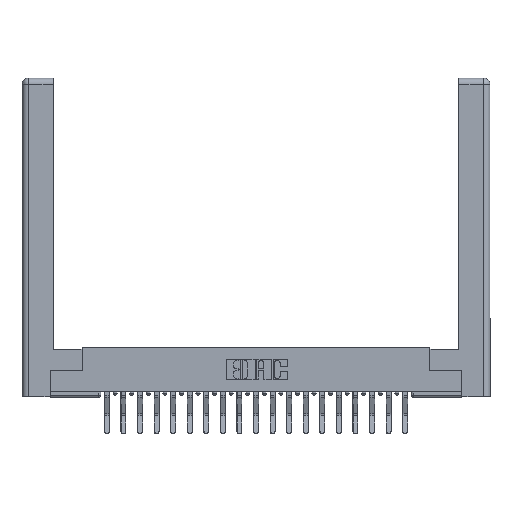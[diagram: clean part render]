
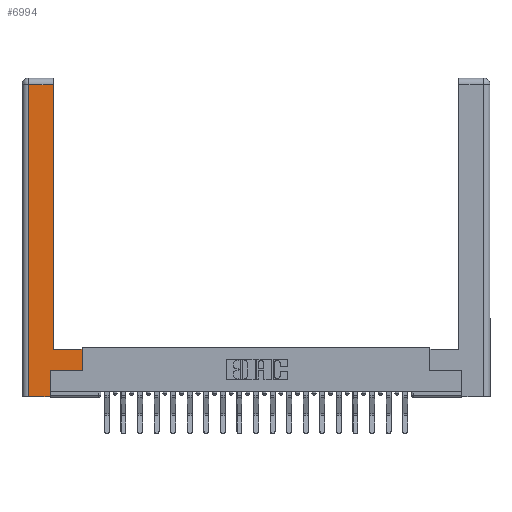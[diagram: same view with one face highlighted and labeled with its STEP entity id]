
A CAD part, top view. The second image highlights one B-rep face of the part: STEP entity #6994.
In plain terms, the highlighted planar face has unit normal (0, 0, 1).
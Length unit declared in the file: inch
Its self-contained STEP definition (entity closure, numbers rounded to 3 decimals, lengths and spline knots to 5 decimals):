
#736 = CARTESIAN_POINT ( 'NONE',  ( 0.565, 0.245, 0. ) ) ;
#1228 = VECTOR ( 'NONE', #2100, 39.37008 ) ;
#1579 = CARTESIAN_POINT ( 'NONE',  ( 0.0615, 2.94, 0. ) ) ;
#1659 = AXIS2_PLACEMENT_3D ( 'NONE', #2252, #16117, #19521 ) ;
#1667 = CARTESIAN_POINT ( 'NONE',  ( 0.295, 0.45, 0. ) ) ;
#1779 = VERTEX_POINT ( 'NONE', #20524 ) ;
#2100 = DIRECTION ( 'NONE',  ( 0., 1., 0. ) ) ;
#2252 = CARTESIAN_POINT ( 'NONE',  ( 0., 0., 0. ) ) ;
#2592 = LINE ( 'NONE', #6267, #15879 ) ;
#3101 = CARTESIAN_POINT ( 'NONE',  ( 0.295, 2.94, 0. ) ) ;
#3472 = DIRECTION ( 'NONE',  ( -1., 0., 0. ) ) ;
#4064 = CARTESIAN_POINT ( 'NONE',  ( 0.565, 0.45, 0. ) ) ;
#4381 = EDGE_CURVE ( 'NONE', #16245, #14861, #12408, .T. ) ;
#4426 = LINE ( 'NONE', #10451, #22373 ) ;
#5362 = VECTOR ( 'NONE', #15289, 39.37008 ) ;
#5821 = DIRECTION ( 'NONE',  ( 0., 1., 0. ) ) ;
#5890 = VECTOR ( 'NONE', #5821, 39.37008 ) ;
#5958 = VECTOR ( 'NONE', #19146, 39.37008 ) ;
#6267 = CARTESIAN_POINT ( 'NONE',  ( 0.0615, 0., 0. ) ) ;
#6269 = VERTEX_POINT ( 'NONE', #3101 ) ;
#6994 = ADVANCED_FACE ( 'NONE', ( #21764 ), #12651, .F. ) ;
#8151 = ORIENTED_EDGE ( 'NONE', *, *, #16688, .T. ) ;
#8344 = LINE ( 'NONE', #736, #18120 ) ;
#9916 = LINE ( 'NONE', #14165, #1228 ) ;
#10451 = CARTESIAN_POINT ( 'NONE',  ( 0.0615, 2.94, 0. ) ) ;
#10456 = DIRECTION ( 'NONE',  ( -1., 0., 0. ) ) ;
#10518 = CARTESIAN_POINT ( 'NONE',  ( 0.295, 0.45, 0. ) ) ;
#11649 = ORIENTED_EDGE ( 'NONE', *, *, #18595, .T. ) ;
#12361 = ORIENTED_EDGE ( 'NONE', *, *, #20280, .T. ) ;
#12408 = LINE ( 'NONE', #4064, #5890 ) ;
#12465 = VERTEX_POINT ( 'NONE', #12523 ) ;
#12523 = CARTESIAN_POINT ( 'NONE',  ( 0.0615, 0., 0. ) ) ;
#12590 = EDGE_CURVE ( 'NONE', #16413, #16245, #8344, .T. ) ;
#12651 = PLANE ( 'NONE',  #1659 ) ;
#13874 = LINE ( 'NONE', #1667, #21977 ) ;
#14165 = CARTESIAN_POINT ( 'NONE',  ( 0.265, 0.245, 0. ) ) ;
#14385 = EDGE_LOOP ( 'NONE', ( #8151, #12361, #11649, #19383, #17170, #17784, #17348, #18415 ) ) ;
#14861 = VERTEX_POINT ( 'NONE', #21602 ) ;
#15128 = EDGE_CURVE ( 'NONE', #14861, #22238, #13874, .T. ) ;
#15289 = DIRECTION ( 'NONE',  ( 0., 1., 0. ) ) ;
#15859 = CARTESIAN_POINT ( 'NONE',  ( 0.265, 0.245, 0. ) ) ;
#15879 = VECTOR ( 'NONE', #17947, 39.37008 ) ;
#16117 = DIRECTION ( 'NONE',  ( 0., 0., -1. ) ) ;
#16245 = VERTEX_POINT ( 'NONE', #22091 ) ;
#16277 = LINE ( 'NONE', #20738, #5958 ) ;
#16413 = VERTEX_POINT ( 'NONE', #15859 ) ;
#16688 = EDGE_CURVE ( 'NONE', #22238, #6269, #19211, .T. ) ;
#16985 = VERTEX_POINT ( 'NONE', #1579 ) ;
#17170 = ORIENTED_EDGE ( 'NONE', *, *, #19042, .T. ) ;
#17348 = ORIENTED_EDGE ( 'NONE', *, *, #4381, .T. ) ;
#17784 = ORIENTED_EDGE ( 'NONE', *, *, #12590, .T. ) ;
#17947 = DIRECTION ( 'NONE',  ( 0., -1., 0. ) ) ;
#18120 = VECTOR ( 'NONE', #19844, 39.37008 ) ;
#18415 = ORIENTED_EDGE ( 'NONE', *, *, #15128, .T. ) ;
#18595 = EDGE_CURVE ( 'NONE', #16985, #12465, #2592, .T. ) ;
#19042 = EDGE_CURVE ( 'NONE', #1779, #16413, #9916, .T. ) ;
#19146 = DIRECTION ( 'NONE',  ( 1., 0., 0. ) ) ;
#19211 = LINE ( 'NONE', #22190, #5362 ) ;
#19383 = ORIENTED_EDGE ( 'NONE', *, *, #22236, .T. ) ;
#19521 = DIRECTION ( 'NONE',  ( -1., 0., 0. ) ) ;
#19844 = DIRECTION ( 'NONE',  ( 1., 0., 0. ) ) ;
#20280 = EDGE_CURVE ( 'NONE', #6269, #16985, #4426, .T. ) ;
#20524 = CARTESIAN_POINT ( 'NONE',  ( 0.265, 0., 0. ) ) ;
#20738 = CARTESIAN_POINT ( 'NONE',  ( 0.265, 0., 0. ) ) ;
#21602 = CARTESIAN_POINT ( 'NONE',  ( 0.565, 0.45, 0. ) ) ;
#21764 = FACE_OUTER_BOUND ( 'NONE', #14385, .T. ) ;
#21977 = VECTOR ( 'NONE', #10456, 39.37008 ) ;
#22091 = CARTESIAN_POINT ( 'NONE',  ( 0.565, 0.245, 0. ) ) ;
#22190 = CARTESIAN_POINT ( 'NONE',  ( 0.295, 3., 0. ) ) ;
#22236 = EDGE_CURVE ( 'NONE', #12465, #1779, #16277, .T. ) ;
#22238 = VERTEX_POINT ( 'NONE', #10518 ) ;
#22373 = VECTOR ( 'NONE', #3472, 39.37008 ) ;
